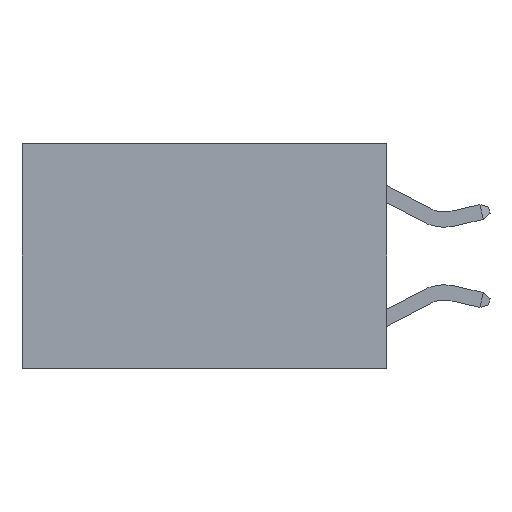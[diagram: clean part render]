
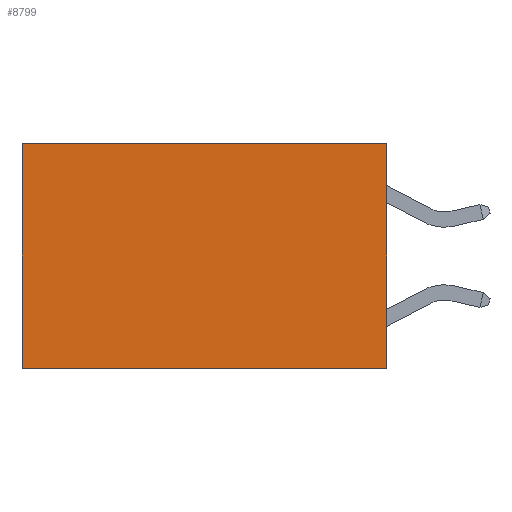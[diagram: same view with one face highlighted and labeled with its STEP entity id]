
A CAD part, left-side view. The second image highlights one B-rep face of the part: STEP entity #8799.
In plain terms, the highlighted planar face has unit normal (-1, 0, 0).
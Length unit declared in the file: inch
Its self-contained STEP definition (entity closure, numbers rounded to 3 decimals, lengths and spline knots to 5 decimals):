
#553 = ORIENTED_EDGE ( 'NONE', *, *, #15229, .T. ) ;
#1207 = CARTESIAN_POINT ( 'NONE',  ( 0.2625, 0., 0. ) ) ;
#1240 = VERTEX_POINT ( 'NONE', #10967 ) ;
#1969 = ORIENTED_EDGE ( 'NONE', *, *, #13348, .F. ) ;
#2690 = VECTOR ( 'NONE', #14817, 39.37008 ) ;
#3447 = LINE ( 'NONE', #10019, #11756 ) ;
#5452 = PLANE ( 'NONE',  #9133 ) ;
#6169 = LINE ( 'NONE', #16398, #11181 ) ;
#7178 = CARTESIAN_POINT ( 'NONE',  ( 0.2625, 0., 0. ) ) ;
#8318 = ORIENTED_EDGE ( 'NONE', *, *, #16796, .T. ) ;
#8626 = LINE ( 'NONE', #10660, #2690 ) ;
#8799 = ADVANCED_FACE ( 'NONE', ( #12047 ), #5452, .F. ) ;
#8821 = VERTEX_POINT ( 'NONE', #11029 ) ;
#9000 = CARTESIAN_POINT ( 'NONE',  ( 0.2625, 0.6, 0. ) ) ;
#9133 = AXIS2_PLACEMENT_3D ( 'NONE', #1207, #12423, #12486 ) ;
#9254 = EDGE_CURVE ( 'NONE', #16376, #8821, #8626, .T. ) ;
#10009 = EDGE_LOOP ( 'NONE', ( #8318, #1969, #12682, #553 ) ) ;
#10019 = CARTESIAN_POINT ( 'NONE',  ( 0.2625, 0.6, 0. ) ) ;
#10660 = CARTESIAN_POINT ( 'NONE',  ( 0.2625, 0., 0. ) ) ;
#10715 = DIRECTION ( 'NONE',  ( 0., 1., 0. ) ) ;
#10782 = VERTEX_POINT ( 'NONE', #9000 ) ;
#10967 = CARTESIAN_POINT ( 'NONE',  ( 0.2625, 0.6, -0.37 ) ) ;
#11029 = CARTESIAN_POINT ( 'NONE',  ( 0.2625, 0., -0.37 ) ) ;
#11181 = VECTOR ( 'NONE', #15113, 39.37008 ) ;
#11325 = DIRECTION ( 'NONE',  ( 0., 0., -1. ) ) ;
#11570 = VECTOR ( 'NONE', #10715, 39.37008 ) ;
#11756 = VECTOR ( 'NONE', #11325, 39.37008 ) ;
#12047 = FACE_OUTER_BOUND ( 'NONE', #10009, .T. ) ;
#12423 = DIRECTION ( 'NONE',  ( 1., 0., 0. ) ) ;
#12486 = DIRECTION ( 'NONE',  ( 0., 0., -1. ) ) ;
#12639 = LINE ( 'NONE', #13464, #11570 ) ;
#12682 = ORIENTED_EDGE ( 'NONE', *, *, #9254, .F. ) ;
#13348 = EDGE_CURVE ( 'NONE', #8821, #1240, #6169, .T. ) ;
#13464 = CARTESIAN_POINT ( 'NONE',  ( 0.2625, 0., 0. ) ) ;
#14817 = DIRECTION ( 'NONE',  ( 0., 0., -1. ) ) ;
#15113 = DIRECTION ( 'NONE',  ( 0., 1., 0. ) ) ;
#15229 = EDGE_CURVE ( 'NONE', #16376, #10782, #12639, .T. ) ;
#16376 = VERTEX_POINT ( 'NONE', #7178 ) ;
#16398 = CARTESIAN_POINT ( 'NONE',  ( 0.2625, 0., -0.37 ) ) ;
#16796 = EDGE_CURVE ( 'NONE', #10782, #1240, #3447, .T. ) ;
